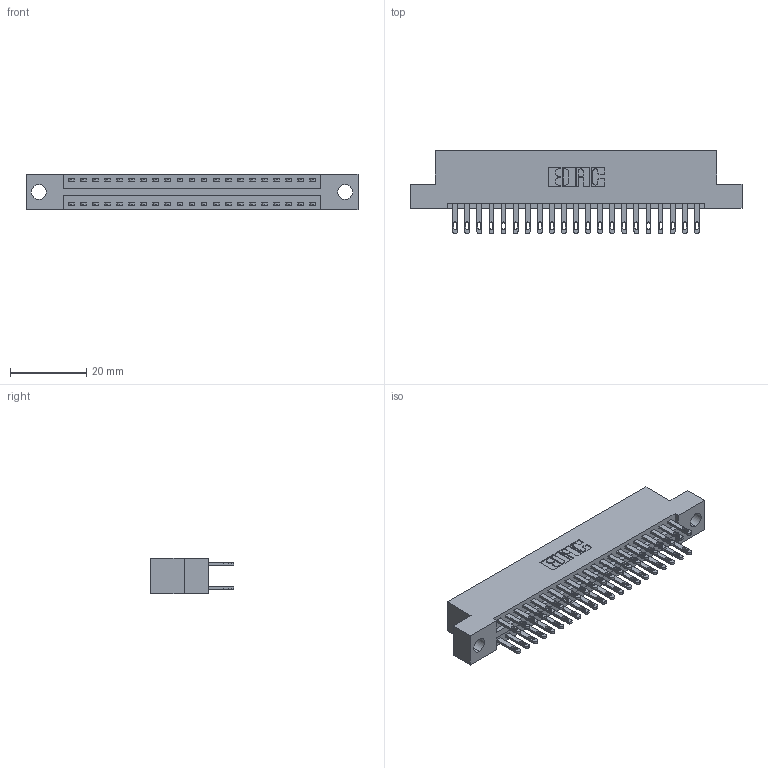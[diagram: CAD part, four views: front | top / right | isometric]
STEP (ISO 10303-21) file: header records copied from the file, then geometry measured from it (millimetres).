
FILE_DESCRIPTION (( 'STEP AP203' ), '1' );
FILE_NAME ('346-042-500-204.STEP', '2022-05-20T03:24:23', ( '' ), ( '' ), 'SwSTEP 2.0', 'SolidWorks 2020', '' );
FILE_SCHEMA (( 'CONFIG_CONTROL_DESIGN' ));
Length unit declared in the file: inch
Products named in the file (3): 345-292-001_345-293-100; 346-042-500-204; 346 Part_Flush Mounting Lugs - 0.156 Dia-TH
Assembly tree (43 placements, depth 2):
  346-042-500-204
    346 Part_Flush Mounting Lugs - 0.156 Dia-TH
    345-292-001_345-293-100  x42
Bounding box: 87.25 x 21.84 x 9.4 mm (x, y, z)
Volume: 8367.2 mm3; surface area: 11458.6 mm2
Topology: 43 solids, 43 shells, 2152 faces, 6539 edges, 4358 vertices
Faces by surface type: plane 1308, cylinder 844
Entity records: 16881 total; most frequent: CARTESIAN_POINT 2814, ORIENTED_EDGE 2746, DIRECTION 2533, EDGE_CURVE 1373, LINE 1153, VECTOR 1153, VERTEX_POINT 914, AXIS2_PLACEMENT_3D 690
